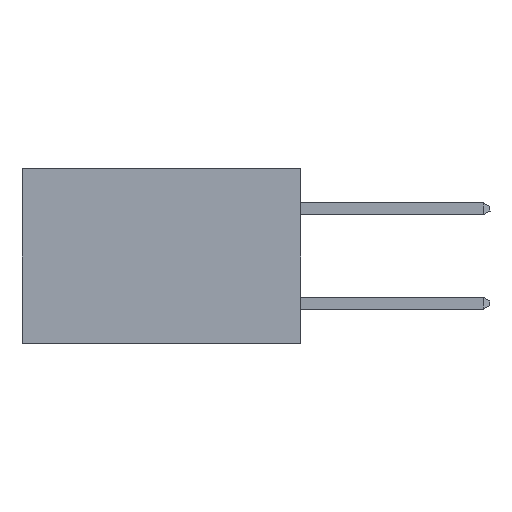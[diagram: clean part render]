
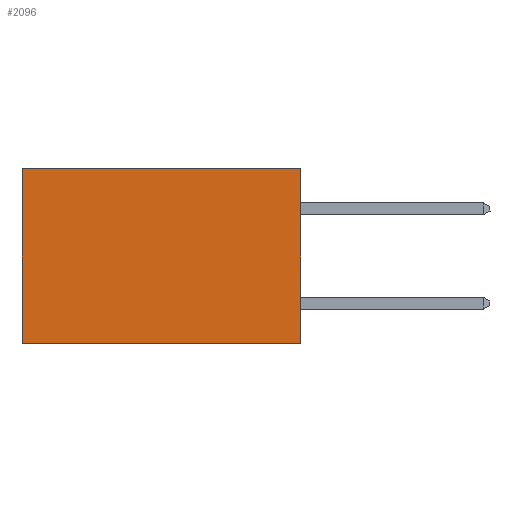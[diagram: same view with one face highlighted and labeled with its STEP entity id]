
A CAD part, left-side view. The second image highlights one B-rep face of the part: STEP entity #2096.
In plain terms, the highlighted planar face has unit normal (-1, 0, 0).
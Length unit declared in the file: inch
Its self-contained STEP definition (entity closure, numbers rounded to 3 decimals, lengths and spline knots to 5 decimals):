
#150 = ORIENTED_EDGE ( 'NONE', *, *, #10505, .F. ) ;
#288 = CARTESIAN_POINT ( 'NONE',  ( 0.277, 0., -0.37 ) ) ;
#609 = CARTESIAN_POINT ( 'NONE',  ( 0.277, 0., 0. ) ) ;
#1013 = FACE_OUTER_BOUND ( 'NONE', #20179, .T. ) ;
#1092 = EDGE_CURVE ( 'NONE', #20585, #7987, #7825, .T. ) ;
#1139 = CARTESIAN_POINT ( 'NONE',  ( 0.277, 0.59, -0.37 ) ) ;
#1421 = LINE ( 'NONE', #20416, #19705 ) ;
#2096 = ADVANCED_FACE ( 'NONE', ( #1013 ), #8433, .F. ) ;
#3957 = ORIENTED_EDGE ( 'NONE', *, *, #20466, .F. ) ;
#6134 = ORIENTED_EDGE ( 'NONE', *, *, #16856, .T. ) ;
#7381 = VECTOR ( 'NONE', #13611, 39.37008 ) ;
#7825 = LINE ( 'NONE', #17259, #21937 ) ;
#7987 = VERTEX_POINT ( 'NONE', #1139 ) ;
#8433 = PLANE ( 'NONE',  #16879 ) ;
#9421 = CARTESIAN_POINT ( 'NONE',  ( 0.277, 0., -0.37 ) ) ;
#10505 = EDGE_CURVE ( 'NONE', #13237, #19316, #1421, .T. ) ;
#10703 = DIRECTION ( 'NONE',  ( 0., 0., -1. ) ) ;
#11977 = DIRECTION ( 'NONE',  ( 0., 1., 0. ) ) ;
#12522 = ORIENTED_EDGE ( 'NONE', *, *, #1092, .T. ) ;
#12790 = VECTOR ( 'NONE', #11977, 39.37008 ) ;
#13101 = DIRECTION ( 'NONE',  ( 0., 0., -1. ) ) ;
#13237 = VERTEX_POINT ( 'NONE', #15948 ) ;
#13382 = LINE ( 'NONE', #609, #12790 ) ;
#13402 = DIRECTION ( 'NONE',  ( 0., 0., -1. ) ) ;
#13611 = DIRECTION ( 'NONE',  ( 0., 1., 0. ) ) ;
#15948 = CARTESIAN_POINT ( 'NONE',  ( 0.277, 0., 0. ) ) ;
#16856 = EDGE_CURVE ( 'NONE', #13237, #20585, #13382, .T. ) ;
#16879 = AXIS2_PLACEMENT_3D ( 'NONE', #9421, #20267, #13402 ) ;
#17259 = CARTESIAN_POINT ( 'NONE',  ( 0.277, 0.59, -0.37 ) ) ;
#17675 = CARTESIAN_POINT ( 'NONE',  ( 0.277, 0.59, 0. ) ) ;
#19316 = VERTEX_POINT ( 'NONE', #22944 ) ;
#19705 = VECTOR ( 'NONE', #13101, 39.37008 ) ;
#20179 = EDGE_LOOP ( 'NONE', ( #12522, #3957, #150, #6134 ) ) ;
#20267 = DIRECTION ( 'NONE',  ( 1., 0., 0. ) ) ;
#20416 = CARTESIAN_POINT ( 'NONE',  ( 0.277, 0., -0.37 ) ) ;
#20466 = EDGE_CURVE ( 'NONE', #19316, #7987, #21505, .T. ) ;
#20585 = VERTEX_POINT ( 'NONE', #17675 ) ;
#21505 = LINE ( 'NONE', #288, #7381 ) ;
#21937 = VECTOR ( 'NONE', #10703, 39.37008 ) ;
#22944 = CARTESIAN_POINT ( 'NONE',  ( 0.277, 0., -0.37 ) ) ;
